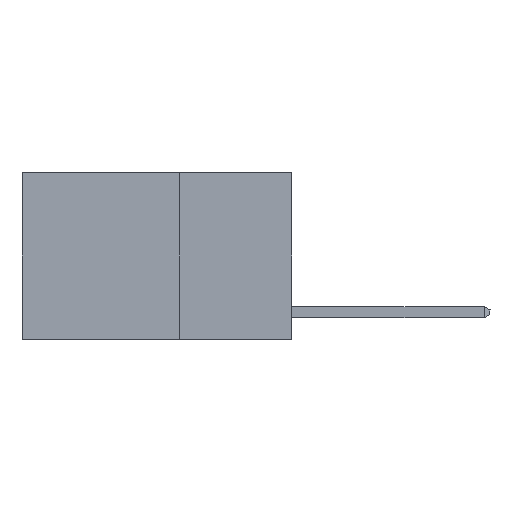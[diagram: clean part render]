
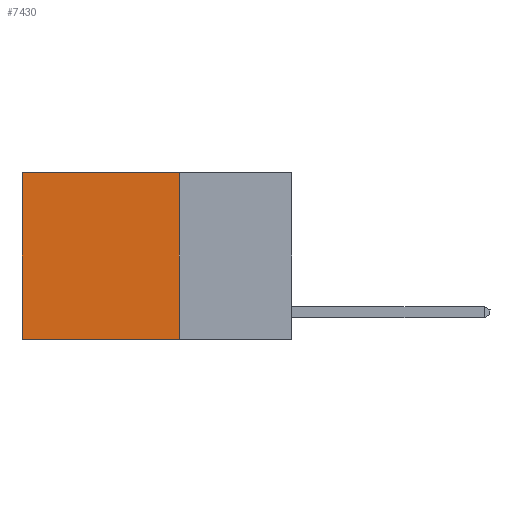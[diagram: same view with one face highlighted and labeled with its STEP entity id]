
A CAD part, left-side view. The second image highlights one B-rep face of the part: STEP entity #7430.
In plain terms, the highlighted planar face has unit normal (-1, 0, 0).
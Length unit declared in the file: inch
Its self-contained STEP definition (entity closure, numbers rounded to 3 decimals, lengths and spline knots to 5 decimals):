
#225 = PLANE ( 'NONE',  #9586 ) ;
#393 = DIRECTION ( 'NONE',  ( 0., 0., -1. ) ) ;
#1012 = FACE_OUTER_BOUND ( 'NONE', #2573, .T. ) ;
#1128 = DIRECTION ( 'NONE',  ( 0., 1., 0. ) ) ;
#1331 = CARTESIAN_POINT ( 'NONE',  ( 0.2625, 0.6, -0.37 ) ) ;
#1406 = LINE ( 'NONE', #8466, #10579 ) ;
#1451 = VERTEX_POINT ( 'NONE', #9559 ) ;
#1482 = EDGE_CURVE ( 'NONE', #4330, #8045, #10230, .T. ) ;
#1855 = EDGE_CURVE ( 'NONE', #3024, #1451, #8959, .T. ) ;
#2064 = DIRECTION ( 'NONE',  ( 1., 0., 0. ) ) ;
#2150 = DIRECTION ( 'NONE',  ( 0., 0., -1. ) ) ;
#2573 = EDGE_LOOP ( 'NONE', ( #6904, #3209, #8570, #11469 ) ) ;
#2599 = CARTESIAN_POINT ( 'NONE',  ( 0.2625, 0.25, 0. ) ) ;
#2646 = CARTESIAN_POINT ( 'NONE',  ( 0.2625, 0.25, -0.37 ) ) ;
#3023 = CARTESIAN_POINT ( 'NONE',  ( 0.2625, 0.25, 0. ) ) ;
#3024 = VERTEX_POINT ( 'NONE', #2599 ) ;
#3209 = ORIENTED_EDGE ( 'NONE', *, *, #1482, .F. ) ;
#3744 = VECTOR ( 'NONE', #1128, 39.37008 ) ;
#4330 = VERTEX_POINT ( 'NONE', #2646 ) ;
#4752 = CARTESIAN_POINT ( 'NONE',  ( 0.2625, 0.25, 0. ) ) ;
#6685 = VECTOR ( 'NONE', #8064, 39.37008 ) ;
#6814 = VECTOR ( 'NONE', #2150, 39.37008 ) ;
#6904 = ORIENTED_EDGE ( 'NONE', *, *, #9348, .T. ) ;
#7430 = ADVANCED_FACE ( 'NONE', ( #1012 ), #225, .F. ) ;
#7435 = CARTESIAN_POINT ( 'NONE',  ( 0.2625, 0.25, 0. ) ) ;
#7964 = EDGE_CURVE ( 'NONE', #3024, #4330, #9375, .T. ) ;
#8045 = VERTEX_POINT ( 'NONE', #1331 ) ;
#8064 = DIRECTION ( 'NONE',  ( 0., 1., 0. ) ) ;
#8271 = DIRECTION ( 'NONE',  ( 0., 0., -1. ) ) ;
#8466 = CARTESIAN_POINT ( 'NONE',  ( 0.2625, 0.6, 0. ) ) ;
#8570 = ORIENTED_EDGE ( 'NONE', *, *, #7964, .F. ) ;
#8789 = CARTESIAN_POINT ( 'NONE',  ( 0.2625, 0.25, -0.37 ) ) ;
#8959 = LINE ( 'NONE', #4752, #6685 ) ;
#9348 = EDGE_CURVE ( 'NONE', #1451, #8045, #1406, .T. ) ;
#9375 = LINE ( 'NONE', #3023, #6814 ) ;
#9559 = CARTESIAN_POINT ( 'NONE',  ( 0.2625, 0.6, 0. ) ) ;
#9586 = AXIS2_PLACEMENT_3D ( 'NONE', #7435, #2064, #8271 ) ;
#10230 = LINE ( 'NONE', #8789, #3744 ) ;
#10579 = VECTOR ( 'NONE', #393, 39.37008 ) ;
#11469 = ORIENTED_EDGE ( 'NONE', *, *, #1855, .T. ) ;
